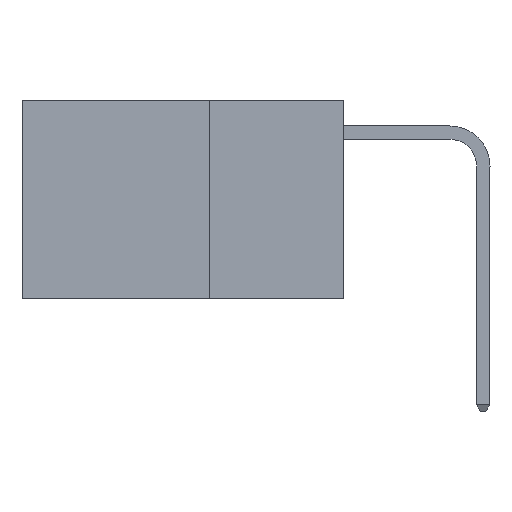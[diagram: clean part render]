
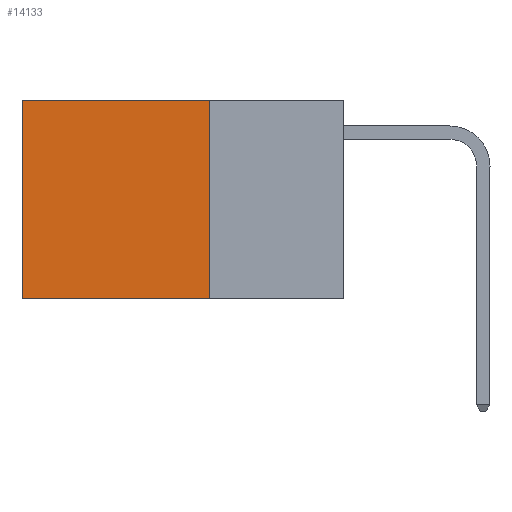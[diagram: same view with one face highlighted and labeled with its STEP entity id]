
A CAD part, left-side view. The second image highlights one B-rep face of the part: STEP entity #14133.
In plain terms, the highlighted planar face has unit normal (-1, 0, 0).
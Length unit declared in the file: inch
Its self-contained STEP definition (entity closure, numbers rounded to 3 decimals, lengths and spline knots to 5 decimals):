
#974 = VERTEX_POINT ( 'NONE', #6882 ) ;
#1008 = DIRECTION ( 'NONE',  ( 0., 0., -1. ) ) ;
#2516 = ORIENTED_EDGE ( 'NONE', *, *, #10572, .T. ) ;
#2703 = VECTOR ( 'NONE', #10072, 39.37008 ) ;
#2718 = CARTESIAN_POINT ( 'NONE',  ( 0.2625, 0.25, 0. ) ) ;
#3752 = EDGE_CURVE ( 'NONE', #13774, #10034, #10019, .T. ) ;
#4259 = CARTESIAN_POINT ( 'NONE',  ( 0.2625, 0.25, -0.37 ) ) ;
#4320 = LINE ( 'NONE', #5411, #7720 ) ;
#4918 = DIRECTION ( 'NONE',  ( 1., 0., 0. ) ) ;
#5062 = VERTEX_POINT ( 'NONE', #17378 ) ;
#5411 = CARTESIAN_POINT ( 'NONE',  ( 0.2625, 0.6, 0. ) ) ;
#5636 = CARTESIAN_POINT ( 'NONE',  ( 0.2625, 0.6, 0. ) ) ;
#6004 = VECTOR ( 'NONE', #16684, 39.37008 ) ;
#6882 = CARTESIAN_POINT ( 'NONE',  ( 0.2625, 0.25, -0.37 ) ) ;
#7257 = EDGE_CURVE ( 'NONE', #13774, #974, #10341, .T. ) ;
#7448 = ORIENTED_EDGE ( 'NONE', *, *, #9326, .F. ) ;
#7720 = VECTOR ( 'NONE', #1008, 39.37008 ) ;
#9326 = EDGE_CURVE ( 'NONE', #974, #5062, #13154, .T. ) ;
#10019 = LINE ( 'NONE', #2718, #2703 ) ;
#10034 = VERTEX_POINT ( 'NONE', #5636 ) ;
#10072 = DIRECTION ( 'NONE',  ( 0., 1., 0. ) ) ;
#10341 = LINE ( 'NONE', #15278, #6004 ) ;
#10572 = EDGE_CURVE ( 'NONE', #10034, #5062, #4320, .T. ) ;
#10728 = CARTESIAN_POINT ( 'NONE',  ( 0.2625, 0.25, 0. ) ) ;
#11539 = ORIENTED_EDGE ( 'NONE', *, *, #3752, .T. ) ;
#11583 = CARTESIAN_POINT ( 'NONE',  ( 0.2625, 0.25, 0. ) ) ;
#13031 = AXIS2_PLACEMENT_3D ( 'NONE', #10728, #4918, #14953 ) ;
#13154 = LINE ( 'NONE', #4259, #13594 ) ;
#13594 = VECTOR ( 'NONE', #14291, 39.37008 ) ;
#13774 = VERTEX_POINT ( 'NONE', #11583 ) ;
#14133 = ADVANCED_FACE ( 'NONE', ( #16489 ), #17716, .F. ) ;
#14291 = DIRECTION ( 'NONE',  ( 0., 1., 0. ) ) ;
#14953 = DIRECTION ( 'NONE',  ( 0., 0., -1. ) ) ;
#15278 = CARTESIAN_POINT ( 'NONE',  ( 0.2625, 0.25, 0. ) ) ;
#16489 = FACE_OUTER_BOUND ( 'NONE', #17807, .T. ) ;
#16684 = DIRECTION ( 'NONE',  ( 0., 0., -1. ) ) ;
#17378 = CARTESIAN_POINT ( 'NONE',  ( 0.2625, 0.6, -0.37 ) ) ;
#17716 = PLANE ( 'NONE',  #13031 ) ;
#17807 = EDGE_LOOP ( 'NONE', ( #2516, #7448, #18528, #11539 ) ) ;
#18528 = ORIENTED_EDGE ( 'NONE', *, *, #7257, .F. ) ;
